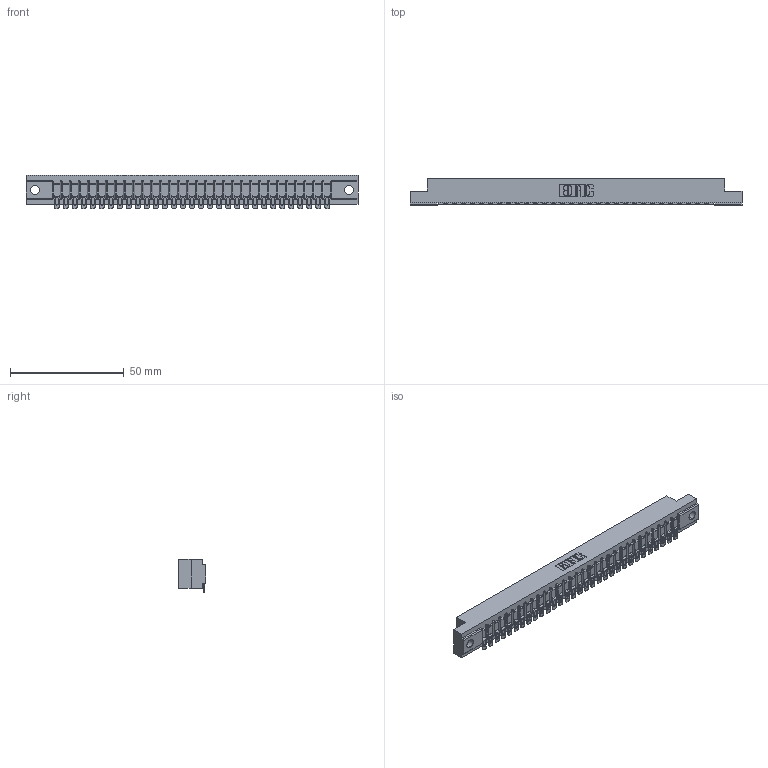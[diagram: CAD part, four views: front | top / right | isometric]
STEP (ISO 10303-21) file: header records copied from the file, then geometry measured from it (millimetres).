
FILE_DESCRIPTION (( 'STEP AP203' ), '1' );
FILE_NAME ('357-031-454-104.STEP', '2020-10-02T04:04:45', ( '' ), ( '' ), 'SwSTEP 2.0', 'SolidWorks 2020', '' );
FILE_SCHEMA (( 'CONFIG_CONTROL_DESIGN' ));
Length unit declared in the file: inch
Products named in the file (3): 307 Part_.156 Dia Mounting Holes; 307-290-002_554; 357-031-454-104
Assembly tree (32 placements, depth 2):
  357-031-454-104
    307 Part_.156 Dia Mounting Holes
    307-290-002_554  x31
Bounding box: 145.85 x 12.01 x 14.52 mm (x, y, z)
Volume: 15430.6 mm3; surface area: 19116.3 mm2
Topology: 32 solids, 32 shells, 2675 faces, 8202 edges, 5380 vertices
Faces by surface type: plane 1510, cylinder 1101, sphere 64
Entity records: 29315 total; most frequent: CARTESIAN_POINT 4948, ORIENTED_EDGE 4936, DIRECTION 4810, EDGE_CURVE 2468, VECTOR 1886, LINE 1886, VERTEX_POINT 1600, AXIS2_PLACEMENT_3D 1462
